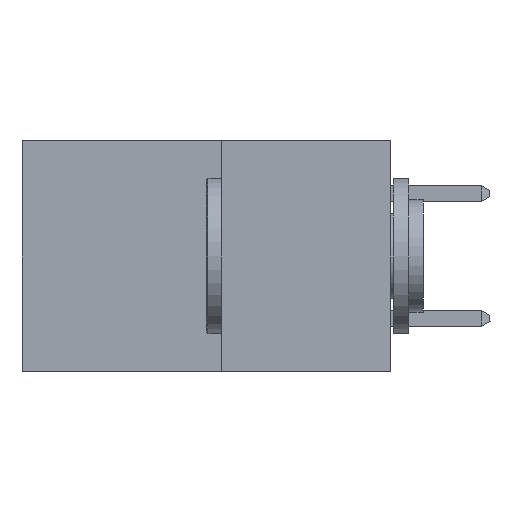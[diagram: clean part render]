
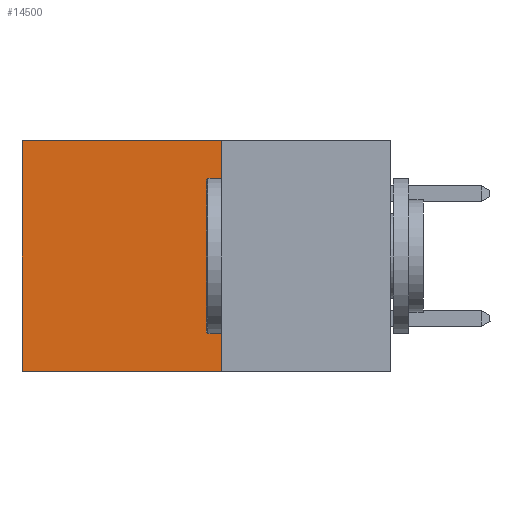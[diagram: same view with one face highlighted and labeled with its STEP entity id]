
A CAD part, left-side view. The second image highlights one B-rep face of the part: STEP entity #14500.
In plain terms, the highlighted planar face has unit normal (-1, 0, 0).
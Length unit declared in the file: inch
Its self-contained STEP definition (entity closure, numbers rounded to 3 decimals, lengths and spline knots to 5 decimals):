
#208 = VECTOR ( 'NONE', #4927, 39.37008 ) ;
#2707 = CARTESIAN_POINT ( 'NONE',  ( 0.277, 0.27, -0.37 ) ) ;
#3077 = ORIENTED_EDGE ( 'NONE', *, *, #7463, .T. ) ;
#3399 = DIRECTION ( 'NONE',  ( 0., 0., -1. ) ) ;
#3697 = CARTESIAN_POINT ( 'NONE',  ( 0.277, 0.59, -0.37 ) ) ;
#4084 = EDGE_CURVE ( 'NONE', #14759, #21841, #19783, .T. ) ;
#4216 = VECTOR ( 'NONE', #3399, 39.37008 ) ;
#4680 = DIRECTION ( 'NONE',  ( 0., 1., 0. ) ) ;
#4927 = DIRECTION ( 'NONE',  ( 0., 0., -1. ) ) ;
#6332 = ORIENTED_EDGE ( 'NONE', *, *, #23379, .F. ) ;
#6529 = AXIS2_PLACEMENT_3D ( 'NONE', #20793, #22697, #11394 ) ;
#6808 = DIRECTION ( 'NONE',  ( 0., 1., 0. ) ) ;
#6995 = CARTESIAN_POINT ( 'NONE',  ( 0.277, 0.27, 0. ) ) ;
#7463 = EDGE_CURVE ( 'NONE', #21841, #12340, #9263, .T. ) ;
#8502 = EDGE_LOOP ( 'NONE', ( #3077, #6332, #21968, #10608 ) ) ;
#9263 = LINE ( 'NONE', #3697, #4216 ) ;
#9479 = PLANE ( 'NONE',  #6529 ) ;
#10263 = LINE ( 'NONE', #18137, #208 ) ;
#10608 = ORIENTED_EDGE ( 'NONE', *, *, #4084, .T. ) ;
#11346 = CARTESIAN_POINT ( 'NONE',  ( 0.277, 0.59, -0.37 ) ) ;
#11394 = DIRECTION ( 'NONE',  ( 0., 0., -1. ) ) ;
#12045 = CARTESIAN_POINT ( 'NONE',  ( 0.277, 0.27, 0. ) ) ;
#12340 = VERTEX_POINT ( 'NONE', #11346 ) ;
#14500 = ADVANCED_FACE ( 'NONE', ( #23077 ), #9479, .F. ) ;
#14759 = VERTEX_POINT ( 'NONE', #12045 ) ;
#15357 = VECTOR ( 'NONE', #6808, 39.37008 ) ;
#15424 = CARTESIAN_POINT ( 'NONE',  ( 0.277, 0.59, 0. ) ) ;
#16196 = EDGE_CURVE ( 'NONE', #14759, #19098, #10263, .T. ) ;
#18123 = VECTOR ( 'NONE', #4680, 39.37008 ) ;
#18137 = CARTESIAN_POINT ( 'NONE',  ( 0.277, 0.27, -0.37 ) ) ;
#19098 = VERTEX_POINT ( 'NONE', #22787 ) ;
#19783 = LINE ( 'NONE', #6995, #15357 ) ;
#20793 = CARTESIAN_POINT ( 'NONE',  ( 0.277, 0.27, -0.37 ) ) ;
#21841 = VERTEX_POINT ( 'NONE', #15424 ) ;
#21968 = ORIENTED_EDGE ( 'NONE', *, *, #16196, .F. ) ;
#22697 = DIRECTION ( 'NONE',  ( 1., 0., 0. ) ) ;
#22787 = CARTESIAN_POINT ( 'NONE',  ( 0.277, 0.27, -0.37 ) ) ;
#23077 = FACE_OUTER_BOUND ( 'NONE', #8502, .T. ) ;
#23193 = LINE ( 'NONE', #2707, #18123 ) ;
#23379 = EDGE_CURVE ( 'NONE', #19098, #12340, #23193, .T. ) ;
